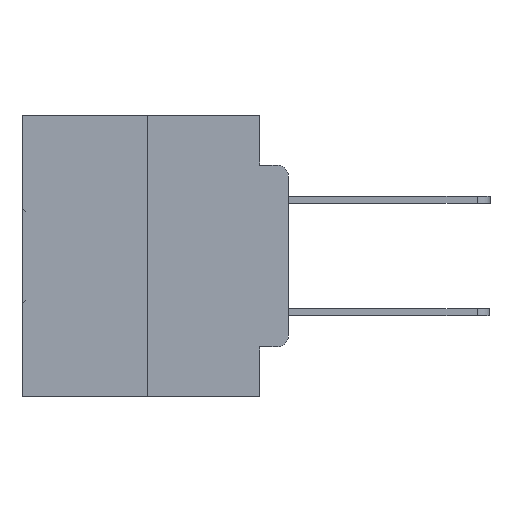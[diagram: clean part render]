
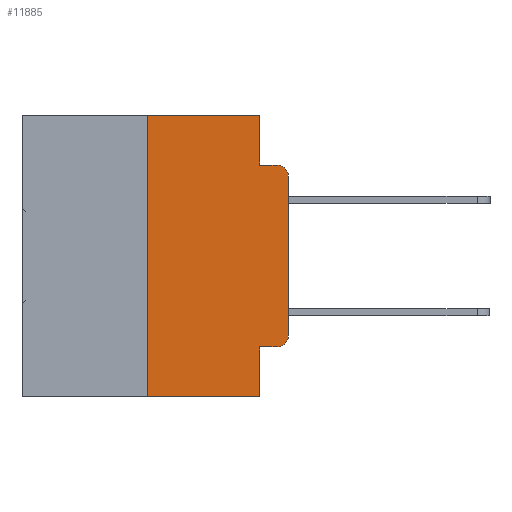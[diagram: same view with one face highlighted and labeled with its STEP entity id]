
A CAD part, left-side view. The second image highlights one B-rep face of the part: STEP entity #11885.
In plain terms, the highlighted planar face has unit normal (-1, 0, 0).
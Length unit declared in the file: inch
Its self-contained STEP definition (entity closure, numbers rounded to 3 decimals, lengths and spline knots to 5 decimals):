
#683 = LINE ( 'NONE', #7425, #32990 ) ;
#1258 = EDGE_CURVE ( 'NONE', #30753, #18396, #2680, .T. ) ;
#1305 = EDGE_CURVE ( 'NONE', #23490, #17918, #14763, .T. ) ;
#1706 = EDGE_CURVE ( 'NONE', #30753, #8564, #23103, .T. ) ;
#2448 = DIRECTION ( 'NONE',  ( 0., 0., -1. ) ) ;
#2495 = CARTESIAN_POINT ( 'NONE',  ( 0., 0.051, -0.0885 ) ) ;
#2680 = LINE ( 'NONE', #6501, #8750 ) ;
#3292 = CARTESIAN_POINT ( 'NONE',  ( 0., 0., -0.1085 ) ) ;
#3681 = VECTOR ( 'NONE', #19405, 39.37008 ) ;
#4000 = DIRECTION ( 'NONE',  ( 0., 0., 1. ) ) ;
#4207 = VECTOR ( 'NONE', #15627, 39.37008 ) ;
#5415 = ORIENTED_EDGE ( 'NONE', *, *, #11963, .F. ) ;
#5808 = EDGE_LOOP ( 'NONE', ( #8237, #26242, #5415, #26235, #7496, #32462, #29056, #27086, #15413, #11861 ) ) ;
#5926 = CARTESIAN_POINT ( 'NONE',  ( 0., 0.02, -0.0885 ) ) ;
#6039 = DIRECTION ( 'NONE',  ( 0., -1., 0. ) ) ;
#6501 = CARTESIAN_POINT ( 'NONE',  ( 0., 0.051, -0.4115 ) ) ;
#6658 = CARTESIAN_POINT ( 'NONE',  ( 0., 0.051, -0.0885 ) ) ;
#7097 = EDGE_CURVE ( 'NONE', #18396, #9461, #25183, .T. ) ;
#7190 = EDGE_CURVE ( 'NONE', #9858, #9257, #22794, .T. ) ;
#7425 = CARTESIAN_POINT ( 'NONE',  ( 0., 0.473, -0.5 ) ) ;
#7496 = ORIENTED_EDGE ( 'NONE', *, *, #9172, .F. ) ;
#7938 = VECTOR ( 'NONE', #2448, 39.37008 ) ;
#8237 = ORIENTED_EDGE ( 'NONE', *, *, #10346, .T. ) ;
#8564 = VERTEX_POINT ( 'NONE', #18053 ) ;
#8750 = VECTOR ( 'NONE', #6039, 39.37008 ) ;
#9172 = EDGE_CURVE ( 'NONE', #24491, #23490, #31796, .T. ) ;
#9257 = VERTEX_POINT ( 'NONE', #5926 ) ;
#9461 = VERTEX_POINT ( 'NONE', #19582 ) ;
#9628 = CARTESIAN_POINT ( 'NONE',  ( 0., 0.051, -0.4115 ) ) ;
#9858 = VERTEX_POINT ( 'NONE', #3292 ) ;
#10346 = EDGE_CURVE ( 'NONE', #9461, #9858, #11084, .T. ) ;
#10403 = CARTESIAN_POINT ( 'NONE',  ( 0., 0.25, -0.5 ) ) ;
#10681 = DIRECTION ( 'NONE',  ( 0., -1., 0. ) ) ;
#11084 = LINE ( 'NONE', #30804, #4207 ) ;
#11227 = DIRECTION ( 'NONE',  ( -1., 0., 0. ) ) ;
#11537 = PLANE ( 'NONE',  #24199 ) ;
#11571 = DIRECTION ( 'NONE',  ( -1., 0., 0. ) ) ;
#11583 = VECTOR ( 'NONE', #10681, 39.37008 ) ;
#11861 = ORIENTED_EDGE ( 'NONE', *, *, #7097, .T. ) ;
#11885 = ADVANCED_FACE ( 'NONE', ( #19736 ), #11537, .F. ) ;
#11963 = EDGE_CURVE ( 'NONE', #17918, #9257, #18117, .T. ) ;
#13523 = VERTEX_POINT ( 'NONE', #10403 ) ;
#14763 = LINE ( 'NONE', #21976, #7938 ) ;
#15413 = ORIENTED_EDGE ( 'NONE', *, *, #1258, .T. ) ;
#15627 = DIRECTION ( 'NONE',  ( 0., 0., 1. ) ) ;
#16639 = DIRECTION ( 'NONE',  ( 0., 0., -1. ) ) ;
#16805 = CARTESIAN_POINT ( 'NONE',  ( 0., 0.25, 0. ) ) ;
#17625 = EDGE_CURVE ( 'NONE', #13523, #24491, #18964, .T. ) ;
#17918 = VERTEX_POINT ( 'NONE', #2495 ) ;
#18053 = CARTESIAN_POINT ( 'NONE',  ( 0., 0.051, -0.5 ) ) ;
#18117 = LINE ( 'NONE', #6658, #3681 ) ;
#18153 = VECTOR ( 'NONE', #4000, 39.37008 ) ;
#18234 = CARTESIAN_POINT ( 'NONE',  ( 0., 0.473, 0. ) ) ;
#18396 = VERTEX_POINT ( 'NONE', #32440 ) ;
#18964 = LINE ( 'NONE', #16805, #18153 ) ;
#19056 = CARTESIAN_POINT ( 'NONE',  ( 0., 0.25, 0. ) ) ;
#19405 = DIRECTION ( 'NONE',  ( 0., -1., 0. ) ) ;
#19582 = CARTESIAN_POINT ( 'NONE',  ( 0., 0., -0.3915 ) ) ;
#19736 = FACE_OUTER_BOUND ( 'NONE', #5808, .T. ) ;
#21756 = CARTESIAN_POINT ( 'NONE',  ( 0., 0.051, 0. ) ) ;
#21976 = CARTESIAN_POINT ( 'NONE',  ( 0., 0.051, 0. ) ) ;
#22794 = CIRCLE ( 'NONE', #30909, 0.02 ) ;
#23103 = LINE ( 'NONE', #21756, #29816 ) ;
#23490 = VERTEX_POINT ( 'NONE', #24773 ) ;
#24000 = DIRECTION ( 'NONE',  ( 0., 0., -1. ) ) ;
#24199 = AXIS2_PLACEMENT_3D ( 'NONE', #29288, #31803, #16639 ) ;
#24491 = VERTEX_POINT ( 'NONE', #19056 ) ;
#24773 = CARTESIAN_POINT ( 'NONE',  ( 0., 0.051, 0. ) ) ;
#25183 = CIRCLE ( 'NONE', #25863, 0.02 ) ;
#25863 = AXIS2_PLACEMENT_3D ( 'NONE', #26469, #11227, #29005 ) ;
#26235 = ORIENTED_EDGE ( 'NONE', *, *, #1305, .F. ) ;
#26242 = ORIENTED_EDGE ( 'NONE', *, *, #7190, .T. ) ;
#26307 = EDGE_CURVE ( 'NONE', #13523, #8564, #683, .T. ) ;
#26469 = CARTESIAN_POINT ( 'NONE',  ( 0., 0.02, -0.3915 ) ) ;
#26787 = CARTESIAN_POINT ( 'NONE',  ( 0., 0.02, -0.1085 ) ) ;
#27086 = ORIENTED_EDGE ( 'NONE', *, *, #1706, .F. ) ;
#27836 = DIRECTION ( 'NONE',  ( 0., -1., 0. ) ) ;
#29005 = DIRECTION ( 'NONE',  ( 0., 0., -1. ) ) ;
#29056 = ORIENTED_EDGE ( 'NONE', *, *, #26307, .T. ) ;
#29288 = CARTESIAN_POINT ( 'NONE',  ( 0., 0.473, 0. ) ) ;
#29319 = DIRECTION ( 'NONE',  ( 0., 0., -1. ) ) ;
#29816 = VECTOR ( 'NONE', #24000, 39.37008 ) ;
#30753 = VERTEX_POINT ( 'NONE', #9628 ) ;
#30804 = CARTESIAN_POINT ( 'NONE',  ( 0., 0., 0. ) ) ;
#30909 = AXIS2_PLACEMENT_3D ( 'NONE', #26787, #11571, #29319 ) ;
#31796 = LINE ( 'NONE', #18234, #11583 ) ;
#31803 = DIRECTION ( 'NONE',  ( 1., 0., 0. ) ) ;
#32440 = CARTESIAN_POINT ( 'NONE',  ( 0., 0.02, -0.4115 ) ) ;
#32462 = ORIENTED_EDGE ( 'NONE', *, *, #17625, .F. ) ;
#32990 = VECTOR ( 'NONE', #27836, 39.37008 ) ;
